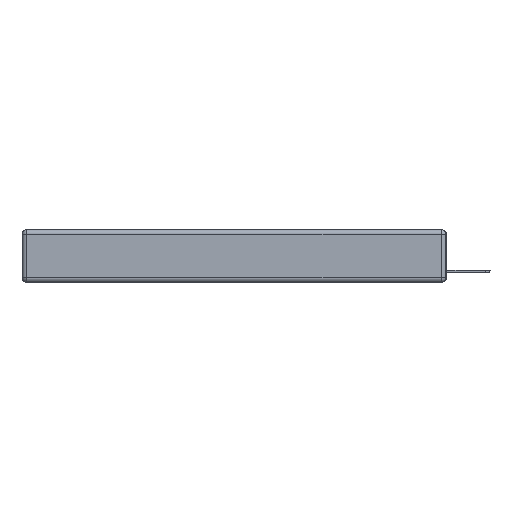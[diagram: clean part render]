
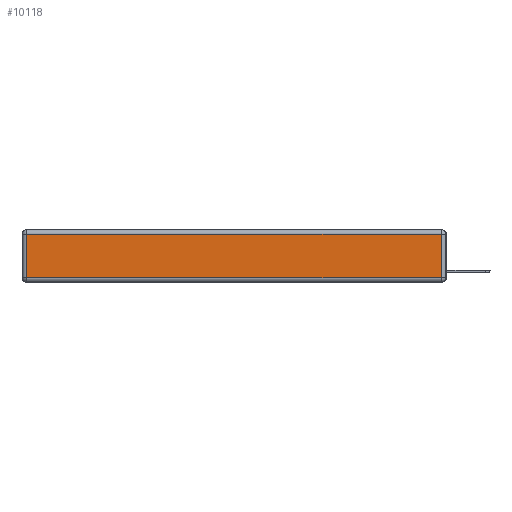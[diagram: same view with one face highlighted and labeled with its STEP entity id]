
A CAD part, left-side view. The second image highlights one B-rep face of the part: STEP entity #10118.
In plain terms, the highlighted planar face has unit normal (-1, 0, 0).
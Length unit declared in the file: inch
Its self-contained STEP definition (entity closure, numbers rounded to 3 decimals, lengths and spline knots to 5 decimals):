
#1206 = LINE ( 'NONE', #1398, #2439 ) ;
#1263 = VECTOR ( 'NONE', #10705, 39.37008 ) ;
#1398 = CARTESIAN_POINT ( 'NONE',  ( 0., 0., -0.313 ) ) ;
#1988 = VERTEX_POINT ( 'NONE', #15497 ) ;
#2439 = VECTOR ( 'NONE', #2899, 39.37008 ) ;
#2456 = VERTEX_POINT ( 'NONE', #14271 ) ;
#2899 = DIRECTION ( 'NONE',  ( 0., -1., 0. ) ) ;
#3107 = EDGE_CURVE ( 'NONE', #2456, #7499, #1206, .T. ) ;
#3802 = VECTOR ( 'NONE', #19163, 39.37008 ) ;
#3944 = LINE ( 'NONE', #13086, #3802 ) ;
#6040 = VERTEX_POINT ( 'NONE', #17311 ) ;
#6167 = LINE ( 'NONE', #13827, #19026 ) ;
#6268 = EDGE_CURVE ( 'NONE', #6040, #2456, #13423, .T. ) ;
#6397 = FACE_OUTER_BOUND ( 'NONE', #16141, .T. ) ;
#7018 = EDGE_CURVE ( 'NONE', #7499, #1988, #3944, .T. ) ;
#7499 = VERTEX_POINT ( 'NONE', #9863 ) ;
#9018 = ORIENTED_EDGE ( 'NONE', *, *, #7018, .T. ) ;
#9279 = AXIS2_PLACEMENT_3D ( 'NONE', #18634, #15460, #17423 ) ;
#9863 = CARTESIAN_POINT ( 'NONE',  ( 0., 0.03, -0.313 ) ) ;
#10118 = ADVANCED_FACE ( 'NONE', ( #6397 ), #15661, .T. ) ;
#10705 = DIRECTION ( 'NONE',  ( 0., 0., -1. ) ) ;
#11707 = ORIENTED_EDGE ( 'NONE', *, *, #16299, .T. ) ;
#12966 = ORIENTED_EDGE ( 'NONE', *, *, #3107, .T. ) ;
#13086 = CARTESIAN_POINT ( 'NONE',  ( 0., 0.03, -0.343 ) ) ;
#13423 = LINE ( 'NONE', #15312, #1263 ) ;
#13827 = CARTESIAN_POINT ( 'NONE',  ( 0., 2.75, -0.03 ) ) ;
#14271 = CARTESIAN_POINT ( 'NONE',  ( 0., 2.72, -0.313 ) ) ;
#15312 = CARTESIAN_POINT ( 'NONE',  ( 0., 2.72, -0.343 ) ) ;
#15460 = DIRECTION ( 'NONE',  ( -1., 0., 0. ) ) ;
#15497 = CARTESIAN_POINT ( 'NONE',  ( 0., 0.03, -0.03 ) ) ;
#15661 = PLANE ( 'NONE',  #9279 ) ;
#15701 = ORIENTED_EDGE ( 'NONE', *, *, #6268, .T. ) ;
#16141 = EDGE_LOOP ( 'NONE', ( #12966, #9018, #11707, #15701 ) ) ;
#16299 = EDGE_CURVE ( 'NONE', #1988, #6040, #6167, .T. ) ;
#17311 = CARTESIAN_POINT ( 'NONE',  ( 0., 2.72, -0.03 ) ) ;
#17423 = DIRECTION ( 'NONE',  ( 0., 0., 1. ) ) ;
#18300 = DIRECTION ( 'NONE',  ( 0., 1., 0. ) ) ;
#18634 = CARTESIAN_POINT ( 'NONE',  ( 0., 0., -0.343 ) ) ;
#19026 = VECTOR ( 'NONE', #18300, 39.37008 ) ;
#19163 = DIRECTION ( 'NONE',  ( 0., 0., 1. ) ) ;
